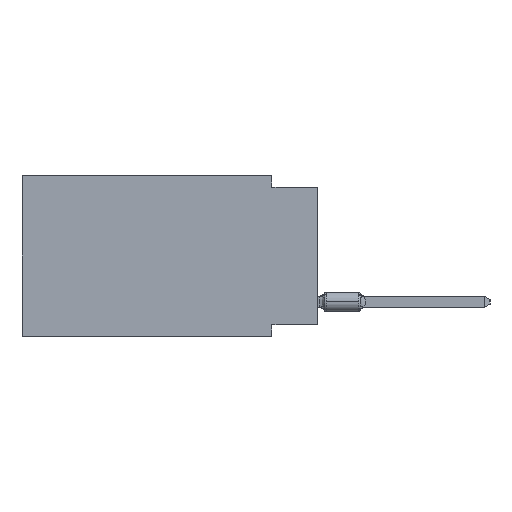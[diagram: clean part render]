
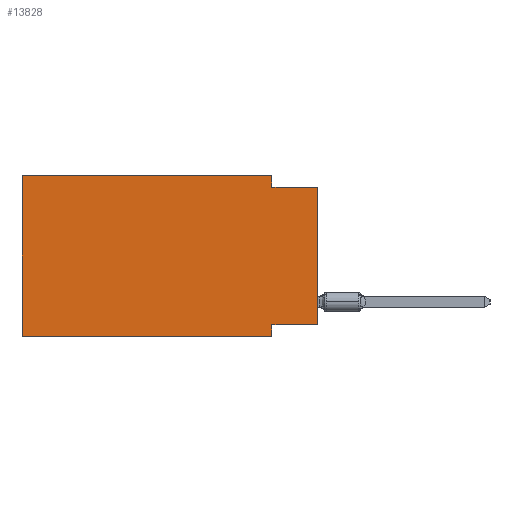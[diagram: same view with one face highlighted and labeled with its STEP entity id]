
A CAD part, left-side view. The second image highlights one B-rep face of the part: STEP entity #13828.
In plain terms, the highlighted planar face has unit normal (-1, 0, 0).
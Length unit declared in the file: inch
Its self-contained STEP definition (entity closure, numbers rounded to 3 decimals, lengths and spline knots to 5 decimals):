
#125 = ORIENTED_EDGE ( 'NONE', *, *, #20015, .F. ) ;
#520 = ORIENTED_EDGE ( 'NONE', *, *, #31874, .F. ) ;
#3272 = EDGE_CURVE ( 'NONE', #5708, #36584, #56572, .T. ) ;
#3714 = CARTESIAN_POINT ( 'NONE',  ( 0., 0.1, -0.35 ) ) ;
#4054 = LINE ( 'NONE', #22117, #45708 ) ;
#5472 = VECTOR ( 'NONE', #32165, 39.37008 ) ;
#5708 = VERTEX_POINT ( 'NONE', #28613 ) ;
#6280 = DIRECTION ( 'NONE',  ( 0., 0., -1. ) ) ;
#6289 = CARTESIAN_POINT ( 'NONE',  ( 0., 0., -0.325 ) ) ;
#6984 = EDGE_CURVE ( 'NONE', #51936, #7982, #43313, .T. ) ;
#7982 = VERTEX_POINT ( 'NONE', #3714 ) ;
#8228 = VECTOR ( 'NONE', #6280, 39.37008 ) ;
#8761 = LINE ( 'NONE', #52697, #13138 ) ;
#9875 = DIRECTION ( 'NONE',  ( 0., -1., 0. ) ) ;
#10155 = ORIENTED_EDGE ( 'NONE', *, *, #28157, .F. ) ;
#10191 = ORIENTED_EDGE ( 'NONE', *, *, #3272, .T. ) ;
#12850 = ORIENTED_EDGE ( 'NONE', *, *, #24146, .F. ) ;
#12872 = DIRECTION ( 'NONE',  ( 0., -1., 0. ) ) ;
#13138 = VECTOR ( 'NONE', #9875, 39.37008 ) ;
#13828 = ADVANCED_FACE ( 'NONE', ( #40557 ), #32500, .F. ) ;
#14383 = CARTESIAN_POINT ( 'NONE',  ( 0., 0.645, 0. ) ) ;
#14434 = DIRECTION ( 'NONE',  ( 1., 0., 0. ) ) ;
#14702 = EDGE_CURVE ( 'NONE', #48525, #52349, #24631, .T. ) ;
#14739 = CARTESIAN_POINT ( 'NONE',  ( 0., 0.1, -0.35 ) ) ;
#15165 = CARTESIAN_POINT ( 'NONE',  ( 0., 0.645, -0.35 ) ) ;
#15183 = LINE ( 'NONE', #6289, #20251 ) ;
#16131 = VERTEX_POINT ( 'NONE', #51920 ) ;
#16668 = CARTESIAN_POINT ( 'NONE',  ( 0., 0.1, 0. ) ) ;
#17505 = DIRECTION ( 'NONE',  ( 0., 0., 1. ) ) ;
#17673 = EDGE_CURVE ( 'NONE', #5708, #56588, #15183, .T. ) ;
#20015 = EDGE_CURVE ( 'NONE', #51936, #16131, #4054, .T. ) ;
#20251 = VECTOR ( 'NONE', #32679, 39.37008 ) ;
#21435 = CARTESIAN_POINT ( 'NONE',  ( 0., 0., -0.025 ) ) ;
#22117 = CARTESIAN_POINT ( 'NONE',  ( 0., 0.645, 0. ) ) ;
#24146 = EDGE_CURVE ( 'NONE', #16131, #48525, #49100, .T. ) ;
#24631 = LINE ( 'NONE', #50179, #8228 ) ;
#25402 = ORIENTED_EDGE ( 'NONE', *, *, #14702, .F. ) ;
#27628 = DIRECTION ( 'NONE',  ( 0., 0., -1. ) ) ;
#28157 = EDGE_CURVE ( 'NONE', #56588, #7982, #32243, .T. ) ;
#28613 = CARTESIAN_POINT ( 'NONE',  ( 0., 0., -0.325 ) ) ;
#30158 = ORIENTED_EDGE ( 'NONE', *, *, #17673, .F. ) ;
#31874 = EDGE_CURVE ( 'NONE', #52349, #36584, #8761, .T. ) ;
#32165 = DIRECTION ( 'NONE',  ( 0., -1., 0. ) ) ;
#32243 = LINE ( 'NONE', #14739, #52900 ) ;
#32500 = PLANE ( 'NONE',  #53944 ) ;
#32679 = DIRECTION ( 'NONE',  ( 0., 1., 0. ) ) ;
#32693 = EDGE_LOOP ( 'NONE', ( #10191, #520, #25402, #12850, #125, #33396, #10155, #30158 ) ) ;
#33396 = ORIENTED_EDGE ( 'NONE', *, *, #6984, .T. ) ;
#34216 = CARTESIAN_POINT ( 'NONE',  ( 0., 0.1, -0.325 ) ) ;
#36584 = VERTEX_POINT ( 'NONE', #21435 ) ;
#39566 = CARTESIAN_POINT ( 'NONE',  ( 0., 0.645, -0.35 ) ) ;
#40557 = FACE_OUTER_BOUND ( 'NONE', #32693, .T. ) ;
#40834 = CARTESIAN_POINT ( 'NONE',  ( 0., 0.645, 0. ) ) ;
#42359 = CARTESIAN_POINT ( 'NONE',  ( 0., 0.1, -0.025 ) ) ;
#43313 = LINE ( 'NONE', #39566, #45202 ) ;
#45202 = VECTOR ( 'NONE', #12872, 39.37008 ) ;
#45708 = VECTOR ( 'NONE', #53127, 39.37008 ) ;
#48496 = CARTESIAN_POINT ( 'NONE',  ( 0., 0., 0. ) ) ;
#48525 = VERTEX_POINT ( 'NONE', #16668 ) ;
#49100 = LINE ( 'NONE', #14383, #5472 ) ;
#50179 = CARTESIAN_POINT ( 'NONE',  ( 0., 0.1, 0. ) ) ;
#51920 = CARTESIAN_POINT ( 'NONE',  ( 0., 0.645, 0. ) ) ;
#51936 = VERTEX_POINT ( 'NONE', #15165 ) ;
#52349 = VERTEX_POINT ( 'NONE', #42359 ) ;
#52697 = CARTESIAN_POINT ( 'NONE',  ( 0., 0., -0.025 ) ) ;
#52900 = VECTOR ( 'NONE', #27628, 39.37008 ) ;
#53127 = DIRECTION ( 'NONE',  ( 0., 0., 1. ) ) ;
#53944 = AXIS2_PLACEMENT_3D ( 'NONE', #40834, #14434, #54059 ) ;
#54024 = VECTOR ( 'NONE', #17505, 39.37008 ) ;
#54059 = DIRECTION ( 'NONE',  ( 0., 0., -1. ) ) ;
#56572 = LINE ( 'NONE', #48496, #54024 ) ;
#56588 = VERTEX_POINT ( 'NONE', #34216 ) ;
